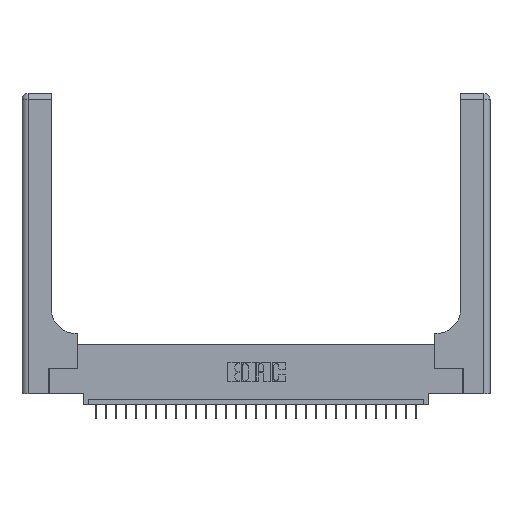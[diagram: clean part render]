
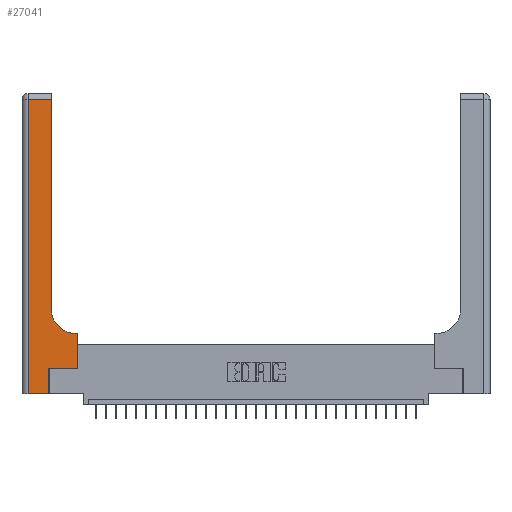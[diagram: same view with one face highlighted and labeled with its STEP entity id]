
A CAD part, top view. The second image highlights one B-rep face of the part: STEP entity #27041.
In plain terms, the highlighted planar face has unit normal (0, 0, 1).
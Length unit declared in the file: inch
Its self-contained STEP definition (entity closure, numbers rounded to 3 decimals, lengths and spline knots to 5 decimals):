
#55 = VECTOR ( 'NONE', #244, 39.37008 ) ;
#244 = DIRECTION ( 'NONE',  ( 0., -1., 0. ) ) ;
#520 = LINE ( 'NONE', #19459, #13352 ) ;
#589 = LINE ( 'NONE', #2971, #25240 ) ;
#796 = VERTEX_POINT ( 'NONE', #13378 ) ;
#1099 = CARTESIAN_POINT ( 'NONE',  ( 0.269, 0., 0.37 ) ) ;
#1805 = CARTESIAN_POINT ( 'NONE',  ( 0.2915, 0.85, 0.37 ) ) ;
#2302 = CARTESIAN_POINT ( 'NONE',  ( 0., 3., 0.37 ) ) ;
#2971 = CARTESIAN_POINT ( 'NONE',  ( 0.269, 0.25, 0.37 ) ) ;
#3223 = CARTESIAN_POINT ( 'NONE',  ( 0.269, 0., 0.37 ) ) ;
#3557 = EDGE_CURVE ( 'NONE', #11432, #5325, #15484, .T. ) ;
#3562 = CARTESIAN_POINT ( 'NONE',  ( 0., 0., 0.37 ) ) ;
#3919 = CARTESIAN_POINT ( 'NONE',  ( 0.5415, 0.85, 0.37 ) ) ;
#4585 = AXIS2_PLACEMENT_3D ( 'NONE', #3919, #20633, #8238 ) ;
#5181 = EDGE_CURVE ( 'NONE', #796, #29154, #589, .T. ) ;
#5209 = DIRECTION ( 'NONE',  ( 1., 0., 0. ) ) ;
#5325 = VERTEX_POINT ( 'NONE', #27457 ) ;
#6016 = EDGE_CURVE ( 'NONE', #5325, #14238, #19446, .T. ) ;
#6186 = CARTESIAN_POINT ( 'NONE',  ( 0.5415, 0.6, 0.37 ) ) ;
#6302 = CARTESIAN_POINT ( 'NONE',  ( 0.5585, 0.6, 0.37 ) ) ;
#7401 = VECTOR ( 'NONE', #22307, 39.37008 ) ;
#7733 = ORIENTED_EDGE ( 'NONE', *, *, #19720, .T. ) ;
#7760 = ORIENTED_EDGE ( 'NONE', *, *, #27981, .T. ) ;
#8238 = DIRECTION ( 'NONE',  ( 1., 0., 0. ) ) ;
#9678 = DIRECTION ( 'NONE',  ( 0., 1., 0. ) ) ;
#9797 = PLANE ( 'NONE',  #19301 ) ;
#10322 = ORIENTED_EDGE ( 'NONE', *, *, #12317, .T. ) ;
#10449 = CARTESIAN_POINT ( 'NONE',  ( 0.06, 3., 0.37 ) ) ;
#11432 = VERTEX_POINT ( 'NONE', #1805 ) ;
#12317 = EDGE_CURVE ( 'NONE', #15048, #796, #17971, .T. ) ;
#12559 = LINE ( 'NONE', #3562, #21852 ) ;
#12621 = EDGE_CURVE ( 'NONE', #29480, #15048, #12559, .T. ) ;
#13352 = VECTOR ( 'NONE', #17704, 39.37008 ) ;
#13378 = CARTESIAN_POINT ( 'NONE',  ( 0.269, 0.25, 0.37 ) ) ;
#13409 = EDGE_CURVE ( 'NONE', #14238, #29480, #26811, .T. ) ;
#13835 = EDGE_CURVE ( 'NONE', #22228, #23061, #520, .T. ) ;
#14238 = VERTEX_POINT ( 'NONE', #24815 ) ;
#14399 = ORIENTED_EDGE ( 'NONE', *, *, #3557, .T. ) ;
#14626 = VECTOR ( 'NONE', #15009, 39.37008 ) ;
#14884 = ORIENTED_EDGE ( 'NONE', *, *, #13835, .T. ) ;
#15009 = DIRECTION ( 'NONE',  ( -1., 0., 0. ) ) ;
#15023 = CARTESIAN_POINT ( 'NONE',  ( 0.5585, 0.25, 0.37 ) ) ;
#15048 = VERTEX_POINT ( 'NONE', #3223 ) ;
#15097 = ORIENTED_EDGE ( 'NONE', *, *, #13409, .T. ) ;
#15322 = CARTESIAN_POINT ( 'NONE',  ( 0.2915, 3., 0.37 ) ) ;
#15484 = LINE ( 'NONE', #15322, #7401 ) ;
#15777 = CARTESIAN_POINT ( 'NONE',  ( 0.5585, 0.25, 0.37 ) ) ;
#15941 = DIRECTION ( 'NONE',  ( 0., 1., 0. ) ) ;
#16647 = ORIENTED_EDGE ( 'NONE', *, *, #5181, .T. ) ;
#17103 = DIRECTION ( 'NONE',  ( -1., 0., 0. ) ) ;
#17704 = DIRECTION ( 'NONE',  ( -1., 0., 0. ) ) ;
#17971 = LINE ( 'NONE', #1099, #24396 ) ;
#18728 = ORIENTED_EDGE ( 'NONE', *, *, #12621, .T. ) ;
#19301 = AXIS2_PLACEMENT_3D ( 'NONE', #2302, #24723, #17103 ) ;
#19446 = LINE ( 'NONE', #24219, #14626 ) ;
#19459 = CARTESIAN_POINT ( 'NONE',  ( 0.2915, 0.6, 0.37 ) ) ;
#19720 = EDGE_CURVE ( 'NONE', #29154, #22228, #24139, .T. ) ;
#19818 = CIRCLE ( 'NONE', #4585, 0.25 ) ;
#20600 = VECTOR ( 'NONE', #15941, 39.37008 ) ;
#20633 = DIRECTION ( 'NONE',  ( 0., 0., -1. ) ) ;
#21852 = VECTOR ( 'NONE', #22222, 39.37008 ) ;
#22178 = FACE_OUTER_BOUND ( 'NONE', #29549, .T. ) ;
#22222 = DIRECTION ( 'NONE',  ( 1., 0., 0. ) ) ;
#22228 = VERTEX_POINT ( 'NONE', #6302 ) ;
#22307 = DIRECTION ( 'NONE',  ( 0., 1., 0. ) ) ;
#23061 = VERTEX_POINT ( 'NONE', #6186 ) ;
#24139 = LINE ( 'NONE', #15777, #20600 ) ;
#24219 = CARTESIAN_POINT ( 'NONE',  ( 0., 2.94, 0.37 ) ) ;
#24396 = VECTOR ( 'NONE', #9678, 39.37008 ) ;
#24723 = DIRECTION ( 'NONE',  ( 0., 0., -1. ) ) ;
#24815 = CARTESIAN_POINT ( 'NONE',  ( 0.06, 2.94, 0.37 ) ) ;
#25240 = VECTOR ( 'NONE', #5209, 39.37008 ) ;
#26239 = CARTESIAN_POINT ( 'NONE',  ( 0.06, 0., 0.37 ) ) ;
#26811 = LINE ( 'NONE', #10449, #55 ) ;
#27041 = ADVANCED_FACE ( 'NONE', ( #22178 ), #9797, .F. ) ;
#27457 = CARTESIAN_POINT ( 'NONE',  ( 0.2915, 2.94, 0.37 ) ) ;
#27499 = ORIENTED_EDGE ( 'NONE', *, *, #6016, .T. ) ;
#27981 = EDGE_CURVE ( 'NONE', #23061, #11432, #19818, .T. ) ;
#29154 = VERTEX_POINT ( 'NONE', #15023 ) ;
#29480 = VERTEX_POINT ( 'NONE', #26239 ) ;
#29549 = EDGE_LOOP ( 'NONE', ( #14399, #27499, #15097, #18728, #10322, #16647, #7733, #14884, #7760 ) ) ;
